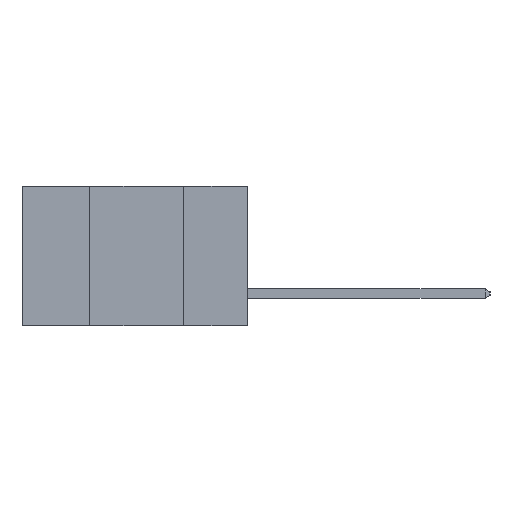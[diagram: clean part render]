
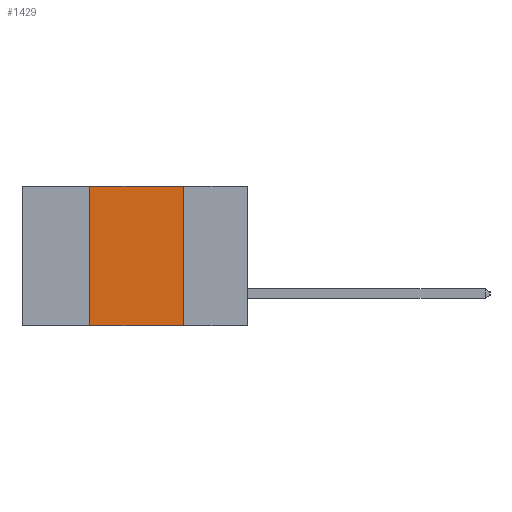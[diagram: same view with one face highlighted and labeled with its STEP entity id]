
A CAD part, left-side view. The second image highlights one B-rep face of the part: STEP entity #1429.
In plain terms, the highlighted planar face has unit normal (-1, 0, 0).
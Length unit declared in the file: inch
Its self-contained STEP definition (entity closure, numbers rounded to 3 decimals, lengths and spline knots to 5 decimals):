
#51 = EDGE_LOOP ( 'NONE', ( #8853, #2894, #9081, #3154 ) ) ;
#310 = VECTOR ( 'NONE', #1881, 39.37008 ) ;
#535 = EDGE_CURVE ( 'NONE', #7968, #2203, #9805, .T. ) ;
#770 = CARTESIAN_POINT ( 'NONE',  ( 0., 0.42, -0.37 ) ) ;
#1270 = EDGE_CURVE ( 'NONE', #7968, #8444, #3057, .T. ) ;
#1429 = ADVANCED_FACE ( 'NONE', ( #9864 ), #7240, .F. ) ;
#1457 = CARTESIAN_POINT ( 'NONE',  ( 0., 0.17, 0. ) ) ;
#1881 = DIRECTION ( 'NONE',  ( 0., 0., 1. ) ) ;
#1897 = EDGE_CURVE ( 'NONE', #8444, #9062, #7284, .T. ) ;
#2203 = VERTEX_POINT ( 'NONE', #7502 ) ;
#2206 = DIRECTION ( 'NONE',  ( 0., 0., -1. ) ) ;
#2243 = CARTESIAN_POINT ( 'NONE',  ( 0., 0.17, -0.37 ) ) ;
#2894 = ORIENTED_EDGE ( 'NONE', *, *, #1897, .F. ) ;
#2986 = EDGE_CURVE ( 'NONE', #9062, #2203, #7607, .T. ) ;
#3057 = LINE ( 'NONE', #770, #310 ) ;
#3154 = ORIENTED_EDGE ( 'NONE', *, *, #535, .T. ) ;
#4008 = VECTOR ( 'NONE', #5342, 39.37008 ) ;
#4875 = CARTESIAN_POINT ( 'NONE',  ( 0., 0.6, -0.37 ) ) ;
#4911 = CARTESIAN_POINT ( 'NONE',  ( 0., 0.42, 0. ) ) ;
#5188 = VECTOR ( 'NONE', #9046, 39.37008 ) ;
#5289 = VECTOR ( 'NONE', #2206, 39.37008 ) ;
#5342 = DIRECTION ( 'NONE',  ( 0., -1., 0. ) ) ;
#5568 = AXIS2_PLACEMENT_3D ( 'NONE', #6893, #6872, #6861 ) ;
#6861 = DIRECTION ( 'NONE',  ( 0., 0., -1. ) ) ;
#6872 = DIRECTION ( 'NONE',  ( 1., 0., 0. ) ) ;
#6893 = CARTESIAN_POINT ( 'NONE',  ( 0., 0.6, 0. ) ) ;
#7240 = PLANE ( 'NONE',  #5568 ) ;
#7284 = LINE ( 'NONE', #9247, #5188 ) ;
#7502 = CARTESIAN_POINT ( 'NONE',  ( 0., 0.17, -0.37 ) ) ;
#7607 = LINE ( 'NONE', #2243, #5289 ) ;
#7968 = VERTEX_POINT ( 'NONE', #8328 ) ;
#8328 = CARTESIAN_POINT ( 'NONE',  ( 0., 0.42, -0.37 ) ) ;
#8444 = VERTEX_POINT ( 'NONE', #4911 ) ;
#8853 = ORIENTED_EDGE ( 'NONE', *, *, #2986, .F. ) ;
#9046 = DIRECTION ( 'NONE',  ( 0., -1., 0. ) ) ;
#9062 = VERTEX_POINT ( 'NONE', #1457 ) ;
#9081 = ORIENTED_EDGE ( 'NONE', *, *, #1270, .F. ) ;
#9247 = CARTESIAN_POINT ( 'NONE',  ( 0., 0.6, 0. ) ) ;
#9805 = LINE ( 'NONE', #4875, #4008 ) ;
#9864 = FACE_OUTER_BOUND ( 'NONE', #51, .T. ) ;
